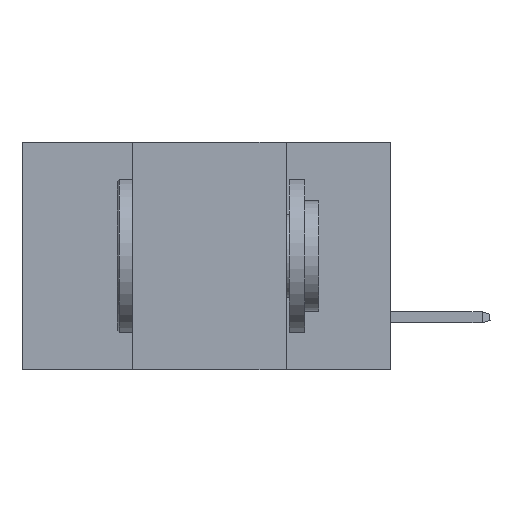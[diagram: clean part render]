
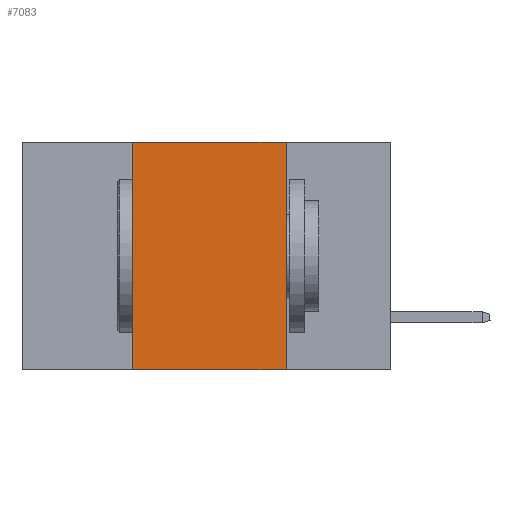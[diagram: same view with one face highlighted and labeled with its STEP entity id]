
A CAD part, left-side view. The second image highlights one B-rep face of the part: STEP entity #7083.
In plain terms, the highlighted planar face has unit normal (-1, 0, 0).
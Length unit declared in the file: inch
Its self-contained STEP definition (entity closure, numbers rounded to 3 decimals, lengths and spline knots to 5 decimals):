
#1825 = VERTEX_POINT ( 'NONE', #21414 ) ;
#2206 = CARTESIAN_POINT ( 'NONE',  ( 0., 0.6, 0. ) ) ;
#2668 = FACE_OUTER_BOUND ( 'NONE', #33907, .T. ) ;
#3237 = LINE ( 'NONE', #32806, #10778 ) ;
#7083 = ADVANCED_FACE ( 'NONE', ( #2668 ), #29759, .F. ) ;
#7635 = CARTESIAN_POINT ( 'NONE',  ( 0., 0.42, 0. ) ) ;
#8460 = CARTESIAN_POINT ( 'NONE',  ( 0., 0.42, 0. ) ) ;
#10547 = VERTEX_POINT ( 'NONE', #26087 ) ;
#10778 = VECTOR ( 'NONE', #25683, 39.37008 ) ;
#10848 = DIRECTION ( 'NONE',  ( 0., 0., -1. ) ) ;
#12191 = VECTOR ( 'NONE', #43125, 39.37008 ) ;
#12342 = ORIENTED_EDGE ( 'NONE', *, *, #41658, .F. ) ;
#13567 = VECTOR ( 'NONE', #10848, 39.37008 ) ;
#17171 = ORIENTED_EDGE ( 'NONE', *, *, #42343, .T. ) ;
#17936 = CARTESIAN_POINT ( 'NONE',  ( 0., 0.17, 0. ) ) ;
#18981 = EDGE_CURVE ( 'NONE', #27520, #43480, #35737, .T. ) ;
#19044 = AXIS2_PLACEMENT_3D ( 'NONE', #2206, #40542, #33130 ) ;
#21414 = CARTESIAN_POINT ( 'NONE',  ( 0., 0.42, -0.37 ) ) ;
#22393 = DIRECTION ( 'NONE',  ( 0., -1., 0. ) ) ;
#22546 = CARTESIAN_POINT ( 'NONE',  ( 0., 0.6, 0. ) ) ;
#22752 = LINE ( 'NONE', #17936, #13567 ) ;
#23519 = ORIENTED_EDGE ( 'NONE', *, *, #18981, .F. ) ;
#25683 = DIRECTION ( 'NONE',  ( 0., -1., 0. ) ) ;
#26087 = CARTESIAN_POINT ( 'NONE',  ( 0., 0.17, -0.37 ) ) ;
#27520 = VERTEX_POINT ( 'NONE', #7635 ) ;
#29759 = PLANE ( 'NONE',  #19044 ) ;
#30624 = LINE ( 'NONE', #8460, #12191 ) ;
#31211 = CARTESIAN_POINT ( 'NONE',  ( 0., 0.17, 0. ) ) ;
#32806 = CARTESIAN_POINT ( 'NONE',  ( 0., 0.6, -0.37 ) ) ;
#33130 = DIRECTION ( 'NONE',  ( 0., 0., -1. ) ) ;
#33907 = EDGE_LOOP ( 'NONE', ( #12342, #23519, #35614, #17171 ) ) ;
#35614 = ORIENTED_EDGE ( 'NONE', *, *, #38906, .F. ) ;
#35737 = LINE ( 'NONE', #22546, #36276 ) ;
#36276 = VECTOR ( 'NONE', #22393, 39.37008 ) ;
#38906 = EDGE_CURVE ( 'NONE', #1825, #27520, #30624, .T. ) ;
#40542 = DIRECTION ( 'NONE',  ( 1., 0., 0. ) ) ;
#41658 = EDGE_CURVE ( 'NONE', #43480, #10547, #22752, .T. ) ;
#42343 = EDGE_CURVE ( 'NONE', #1825, #10547, #3237, .T. ) ;
#43125 = DIRECTION ( 'NONE',  ( 0., 0., 1. ) ) ;
#43480 = VERTEX_POINT ( 'NONE', #31211 ) ;
